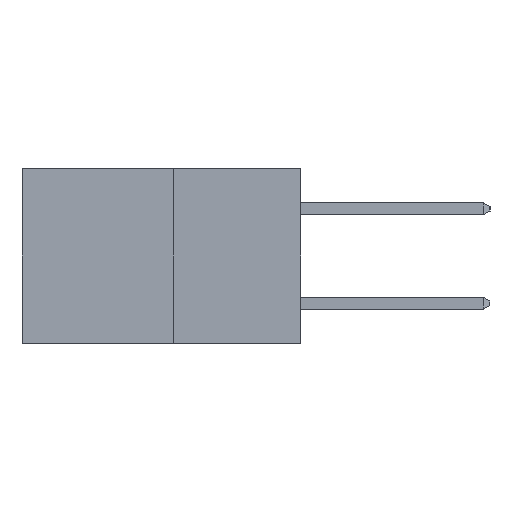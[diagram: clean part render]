
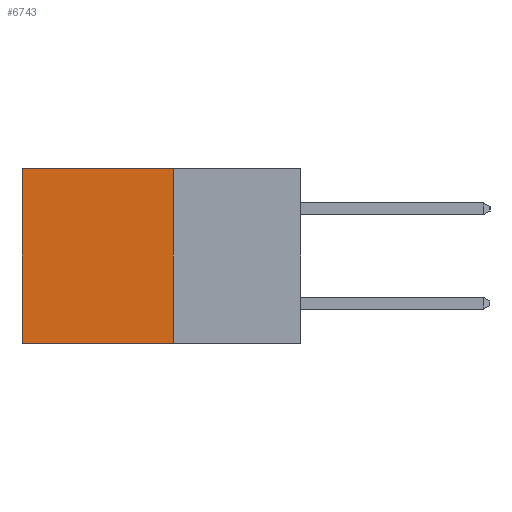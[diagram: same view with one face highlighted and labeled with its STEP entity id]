
A CAD part, left-side view. The second image highlights one B-rep face of the part: STEP entity #6743.
In plain terms, the highlighted planar face has unit normal (-1, 0, 0).
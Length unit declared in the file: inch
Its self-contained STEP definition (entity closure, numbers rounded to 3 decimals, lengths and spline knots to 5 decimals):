
#242 = CARTESIAN_POINT ( 'NONE',  ( 0.277, 0.27, -0.37 ) ) ;
#1677 = EDGE_CURVE ( 'NONE', #8444, #9413, #14469, .T. ) ;
#1894 = DIRECTION ( 'NONE',  ( 0., 0., -1. ) ) ;
#2013 = DIRECTION ( 'NONE',  ( 0., 0., -1. ) ) ;
#2026 = CARTESIAN_POINT ( 'NONE',  ( 0.277, 0.27, -0.37 ) ) ;
#2480 = EDGE_LOOP ( 'NONE', ( #7165, #10018, #13614, #3319 ) ) ;
#3017 = VERTEX_POINT ( 'NONE', #8448 ) ;
#3232 = DIRECTION ( 'NONE',  ( 0., 1., 0. ) ) ;
#3319 = ORIENTED_EDGE ( 'NONE', *, *, #9572, .T. ) ;
#4690 = CARTESIAN_POINT ( 'NONE',  ( 0.277, 0.27, 0. ) ) ;
#5673 = CARTESIAN_POINT ( 'NONE',  ( 0.277, 0.59, -0.37 ) ) ;
#6639 = AXIS2_PLACEMENT_3D ( 'NONE', #14743, #14637, #14597 ) ;
#6743 = ADVANCED_FACE ( 'NONE', ( #9240 ), #14654, .F. ) ;
#6903 = CARTESIAN_POINT ( 'NONE',  ( 0.277, 0.27, 0. ) ) ;
#7155 = VECTOR ( 'NONE', #13366, 39.37008 ) ;
#7165 = ORIENTED_EDGE ( 'NONE', *, *, #1677, .T. ) ;
#8444 = VERTEX_POINT ( 'NONE', #11325 ) ;
#8448 = CARTESIAN_POINT ( 'NONE',  ( 0.277, 0.27, -0.37 ) ) ;
#8851 = VECTOR ( 'NONE', #2013, 39.37008 ) ;
#9034 = EDGE_CURVE ( 'NONE', #13021, #3017, #12262, .T. ) ;
#9240 = FACE_OUTER_BOUND ( 'NONE', #2480, .T. ) ;
#9413 = VERTEX_POINT ( 'NONE', #12427 ) ;
#9572 = EDGE_CURVE ( 'NONE', #13021, #8444, #13052, .T. ) ;
#9765 = VECTOR ( 'NONE', #3232, 39.37008 ) ;
#10018 = ORIENTED_EDGE ( 'NONE', *, *, #11916, .F. ) ;
#11073 = LINE ( 'NONE', #242, #7155 ) ;
#11325 = CARTESIAN_POINT ( 'NONE',  ( 0.277, 0.59, 0. ) ) ;
#11916 = EDGE_CURVE ( 'NONE', #3017, #9413, #11073, .T. ) ;
#12262 = LINE ( 'NONE', #2026, #8851 ) ;
#12427 = CARTESIAN_POINT ( 'NONE',  ( 0.277, 0.59, -0.37 ) ) ;
#13021 = VERTEX_POINT ( 'NONE', #4690 ) ;
#13052 = LINE ( 'NONE', #6903, #9765 ) ;
#13366 = DIRECTION ( 'NONE',  ( 0., 1., 0. ) ) ;
#13614 = ORIENTED_EDGE ( 'NONE', *, *, #9034, .F. ) ;
#14145 = VECTOR ( 'NONE', #1894, 39.37008 ) ;
#14469 = LINE ( 'NONE', #5673, #14145 ) ;
#14597 = DIRECTION ( 'NONE',  ( 0., 0., -1. ) ) ;
#14637 = DIRECTION ( 'NONE',  ( 1., 0., 0. ) ) ;
#14654 = PLANE ( 'NONE',  #6639 ) ;
#14743 = CARTESIAN_POINT ( 'NONE',  ( 0.277, 0.27, -0.37 ) ) ;
